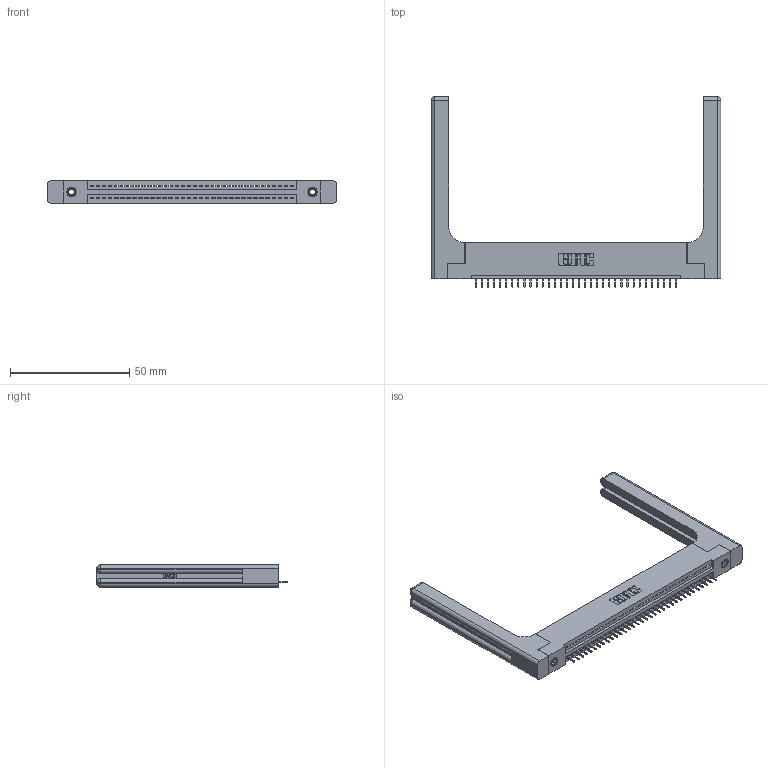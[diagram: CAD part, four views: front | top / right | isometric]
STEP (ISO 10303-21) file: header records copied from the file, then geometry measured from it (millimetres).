
FILE_DESCRIPTION (( 'STEP AP203' ), '1' );
FILE_NAME ('395-034-525-158.STEP', '2020-09-23T22:06:53', ( '' ), ( '' ), 'SwSTEP 2.0', 'SolidWorks 2020', '' );
FILE_SCHEMA (( 'CONFIG_CONTROL_DESIGN' ));
Length unit declared in the file: inch
Products named in the file (5): 345 Part_Flush Mounting Lugs - 0.156 Dia-TH; 395-034-525-158; 345-220-058_345-220-058; 345-250-001_345-250-001-102; 345-292-001_345-293-125
Assembly tree (39 placements, depth 2):
  395-034-525-158
    345 Part_Flush Mounting Lugs - 0.156 Dia-TH
    345-292-001_345-293-125  x34
    345-250-001_345-250-001-102  x2
    345-220-058_345-220-058  x2
Bounding box: 121.39 x 79.68 x 9.4 mm (x, y, z)
Volume: 19830 mm3; surface area: 19783.9 mm2
Topology: 39 solids, 39 shells, 2490 faces, 7127 edges, 4594 vertices
Faces by surface type: plane 1792, cylinder 638, bspline 36, cone 12, sphere 8, torus 4
Entity records: 31922 total; most frequent: CARTESIAN_POINT 6499, ORIENTED_EDGE 5264, DIRECTION 4636, EDGE_CURVE 2632, VECTOR 2276, LINE 2276, VERTEX_POINT 1742, AXIS2_PLACEMENT_3D 1180
